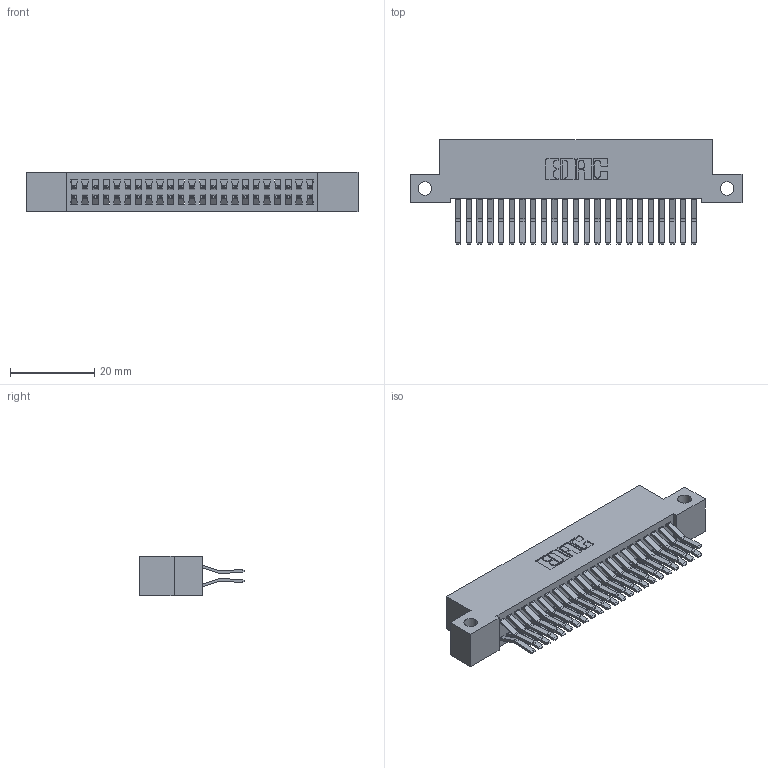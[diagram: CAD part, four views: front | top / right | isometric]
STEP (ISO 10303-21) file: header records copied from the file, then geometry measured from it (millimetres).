
FILE_DESCRIPTION (( 'STEP AP203' ), '1' );
FILE_NAME ('392-046-560-212.STEP', '2019-10-08T00:12:05', ( '' ), ( '' ), 'SwSTEP 2.0', 'SolidWorks 2016', '' );
FILE_SCHEMA (( 'CONFIG_CONTROL_DESIGN' ));
Length unit declared in the file: inch
Products named in the file (3): 342 Part_Side Mount; 345-292-001_560 Tail; 392-046-560-212
Assembly tree (47 placements, depth 2):
  392-046-560-212
    342 Part_Side Mount
    345-292-001_560 Tail  x46
Bounding box: 78.74 x 24.78 x 9.4 mm (x, y, z)
Volume: 7212.9 mm3; surface area: 11837.1 mm2
Topology: 47 solids, 47 shells, 2594 faces, 7705 edges, 5074 vertices
Faces by surface type: plane 1722, cylinder 872
Entity records: 17213 total; most frequent: CARTESIAN_POINT 2874, ORIENTED_EDGE 2810, DIRECTION 2493, EDGE_CURVE 1405, LINE 1273, VECTOR 1273, VERTEX_POINT 934, AXIS2_PLACEMENT_3D 610
